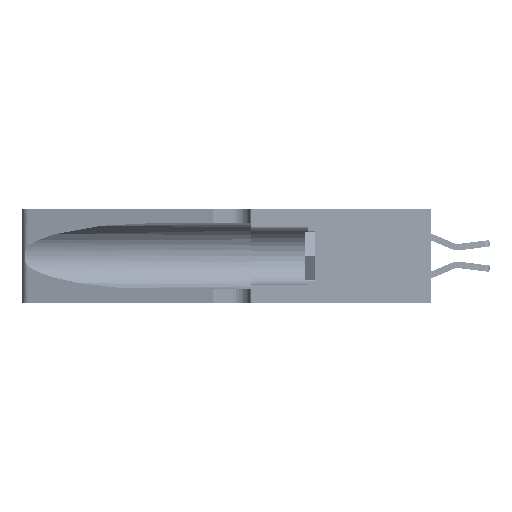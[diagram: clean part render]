
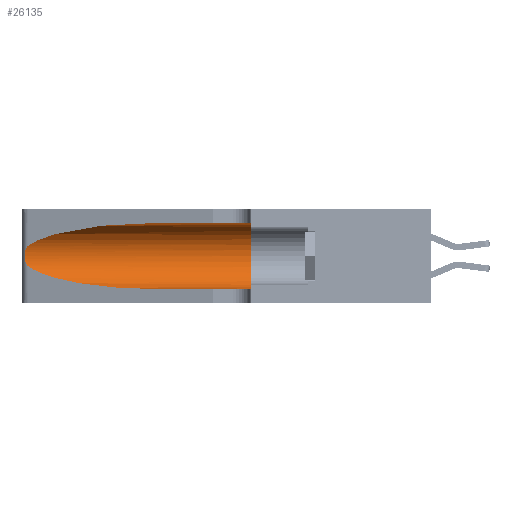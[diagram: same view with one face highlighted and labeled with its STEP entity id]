
A CAD part, left-side view. The second image highlights one B-rep face of the part: STEP entity #26135.
In plain terms, the highlighted cylindrical face has radius 3.308 mm (diameter 6.617 mm), a partial arc.
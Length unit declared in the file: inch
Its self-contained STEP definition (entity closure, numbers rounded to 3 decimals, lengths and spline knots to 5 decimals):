
#650 = CARTESIAN_POINT ( 'NONE',  ( 0.2373, 1.15595, 0.28018 ) ) ;
#911 = CARTESIAN_POINT ( 'NONE',  ( 0.26075, 1.23896, 0.19203 ) ) ;
#1128 = CARTESIAN_POINT ( 'NONE',  ( 0.1305, 1.61858, 0.185 ) ) ;
#1549 = CARTESIAN_POINT ( 'NONE',  ( 0.25487, 1.22718, 0.22369 ) ) ;
#1945 = VERTEX_POINT ( 'NONE', #14002 ) ;
#2865 = CARTESIAN_POINT ( 'NONE',  ( 0.1305, 0.35, 0.05475 ) ) ;
#4366 = DIRECTION ( 'NONE',  ( 0., 0., -1. ) ) ;
#5100 = CARTESIAN_POINT ( 'NONE',  ( 0.26018, 1.23835, 0.19895 ) ) ;
#7176 = ORIENTED_EDGE ( 'NONE', *, *, #41593, .T. ) ;
#7664 = EDGE_LOOP ( 'NONE', ( #7176, #24418, #13960, #9307, #16133, #40132 ) ) ;
#7927 =( BOUNDED_CURVE ( )  B_SPLINE_CURVE ( 3, ( #41032, #44507, #34525, #27306 ),
 .UNSPECIFIED., .F., .F. ) 
 B_SPLINE_CURVE_WITH_KNOTS ( ( 4, 4 ),
 ( 3.44316, 4.71239 ),
 .UNSPECIFIED. ) 
 CURVE ( )  GEOMETRIC_REPRESENTATION_ITEM ( )  RATIONAL_B_SPLINE_CURVE ( ( 1., 0.87, 0.87, 1. ) ) 
 REPRESENTATION_ITEM ( '' )  );
#8252 = CARTESIAN_POINT ( 'NONE',  ( 0.26075, 1.23896, 0.178 ) ) ;
#8406 = CARTESIAN_POINT ( 'NONE',  ( 0.25639, 1.23184, 0.21858 ) ) ;
#8559 = CARTESIAN_POINT ( 'NONE',  ( 0.25639, 1.23186, 0.15144 ) ) ;
#8852 = CARTESIAN_POINT ( 'NONE',  ( 0.1305, 0.35, 0.185 ) ) ;
#9307 = ORIENTED_EDGE ( 'NONE', *, *, #20827, .T. ) ;
#9525 = CYLINDRICAL_SURFACE ( 'NONE', #24399, 0.13025 ) ;
#9622 = CARTESIAN_POINT ( 'NONE',  ( 0.1305, 0.72297, 0.05475 ) ) ;
#11768 = EDGE_CURVE ( 'NONE', #23149, #28576, #24482, .T. ) ;
#12333 = DIRECTION ( 'NONE',  ( 0., 1., 0. ) ) ;
#12676 = VECTOR ( 'NONE', #42101, 39.37008 ) ;
#13960 = ORIENTED_EDGE ( 'NONE', *, *, #37642, .T. ) ;
#13996 = EDGE_CURVE ( 'NONE', #28576, #34873, #18341, .T. ) ;
#14002 = CARTESIAN_POINT ( 'NONE',  ( 0.25487, 1.22718, 0.22369 ) ) ;
#14007 = VECTOR ( 'NONE', #21819, 39.37008 ) ;
#14443 = CARTESIAN_POINT ( 'NONE',  ( 0.1305, 0.72297, 0.31525 ) ) ;
#14993 = CARTESIAN_POINT ( 'NONE',  ( 0.25555, 1.22994, 0.2215 ) ) ;
#15467 = CARTESIAN_POINT ( 'NONE',  ( 0.25854, 1.2359, 0.20912 ) ) ;
#16133 = ORIENTED_EDGE ( 'NONE', *, *, #13996, .F. ) ;
#17205 = LINE ( 'NONE', #29371, #14007 ) ;
#17382 = CARTESIAN_POINT ( 'NONE',  ( 0.1305, 1.61858, 0.31525 ) ) ;
#18341 = CIRCLE ( 'NONE', #44518, 0.13025 ) ;
#20232 = FACE_OUTER_BOUND ( 'NONE', #7664, .T. ) ;
#20827 = EDGE_CURVE ( 'NONE', #44609, #34873, #17205, .T. ) ;
#21228 = CARTESIAN_POINT ( 'NONE',  ( 0.18966, 0.96281, 0.31525 ) ) ;
#21819 = DIRECTION ( 'NONE',  ( 0., -1., 0. ) ) ;
#23149 = VERTEX_POINT ( 'NONE', #31425 ) ;
#24399 = AXIS2_PLACEMENT_3D ( 'NONE', #1128, #35268, #4366 ) ;
#24418 = ORIENTED_EDGE ( 'NONE', *, *, #44302, .T. ) ;
#24482 = LINE ( 'NONE', #17382, #12676 ) ;
#24553 = CARTESIAN_POINT ( 'NONE',  ( 0.25487, 1.22718, 0.22369 ) ) ;
#25109 = CARTESIAN_POINT ( 'NONE',  ( 0.26017, 1.23833, 0.17102 ) ) ;
#25271 = CARTESIAN_POINT ( 'NONE',  ( 0.25787, 1.23484, 0.2124 ) ) ;
#25574 = DIRECTION ( 'NONE',  ( 0., 0., 1. ) ) ;
#25582 = CARTESIAN_POINT ( 'NONE',  ( 0.25856, 1.23593, 0.16098 ) ) ;
#26135 = ADVANCED_FACE ( 'NONE', ( #20232 ), #9525, .F. ) ;
#27306 = CARTESIAN_POINT ( 'NONE',  ( 0.1305, 0.72297, 0.05475 ) ) ;
#28576 = VERTEX_POINT ( 'NONE', #30973 ) ;
#28724 = CARTESIAN_POINT ( 'NONE',  ( 0.25487, 1.22718, 0.14631 ) ) ;
#29189 = CARTESIAN_POINT ( 'NONE',  ( 0.25789, 1.23486, 0.15765 ) ) ;
#29371 = CARTESIAN_POINT ( 'NONE',  ( 0.1305, 1.61858, 0.05475 ) ) ;
#30973 = CARTESIAN_POINT ( 'NONE',  ( 0.1305, 0.35, 0.31525 ) ) ;
#31425 = CARTESIAN_POINT ( 'NONE',  ( 0.1305, 0.72297, 0.31525 ) ) ;
#32787 =( BOUNDED_CURVE ( )  B_SPLINE_CURVE ( 3, ( #14443, #21228, #650, #24553 ),
 .UNSPECIFIED., .F., .T. ) 
 B_SPLINE_CURVE_WITH_KNOTS ( ( 4, 4 ),
 ( 1.5708, 2.84003 ),
 .UNSPECIFIED. ) 
 CURVE ( )  GEOMETRIC_REPRESENTATION_ITEM ( )  RATIONAL_B_SPLINE_CURVE ( ( 1., 0.87, 0.87, 1. ) ) 
 REPRESENTATION_ITEM ( '' )  );
#34525 = CARTESIAN_POINT ( 'NONE',  ( 0.18966, 0.96281, 0.05475 ) ) ;
#34873 = VERTEX_POINT ( 'NONE', #2865 ) ;
#35268 = DIRECTION ( 'NONE',  ( 0., -1., 0. ) ) ;
#36104 = B_SPLINE_CURVE_WITH_KNOTS ( 'NONE', 3,
 ( #1549, #14993, #8406, #25271, #15467, #5100, #911, #8252, #25109, #25582, #29189, #8559, #36123, #28724 ),
 .UNSPECIFIED., .F., .F.,
 ( 4, 2, 2, 2, 2, 2, 4 ),
 ( 0., 0.00027, 0.00053, 0.00107, 0.0016, 0.00187, 0.00214 ),
 .UNSPECIFIED. ) ;
#36123 = CARTESIAN_POINT ( 'NONE',  ( 0.25555, 1.22993, 0.14849 ) ) ;
#37642 = EDGE_CURVE ( 'NONE', #38143, #44609, #7927, .T. ) ;
#38143 = VERTEX_POINT ( 'NONE', #43855 ) ;
#40132 = ORIENTED_EDGE ( 'NONE', *, *, #11768, .F. ) ;
#41032 = CARTESIAN_POINT ( 'NONE',  ( 0.25487, 1.22718, 0.14631 ) ) ;
#41593 = EDGE_CURVE ( 'NONE', #23149, #1945, #32787, .T. ) ;
#42101 = DIRECTION ( 'NONE',  ( 0., -1., 0. ) ) ;
#43855 = CARTESIAN_POINT ( 'NONE',  ( 0.25487, 1.22718, 0.14631 ) ) ;
#44302 = EDGE_CURVE ( 'NONE', #1945, #38143, #36104, .T. ) ;
#44507 = CARTESIAN_POINT ( 'NONE',  ( 0.2373, 1.15595, 0.08982 ) ) ;
#44518 = AXIS2_PLACEMENT_3D ( 'NONE', #8852, #12333, #25574 ) ;
#44609 = VERTEX_POINT ( 'NONE', #9622 ) ;
